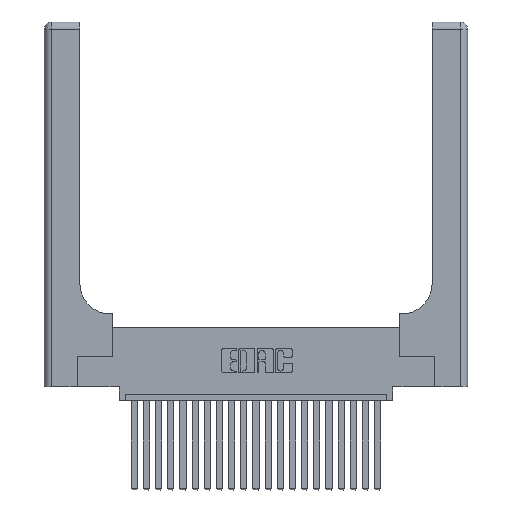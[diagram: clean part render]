
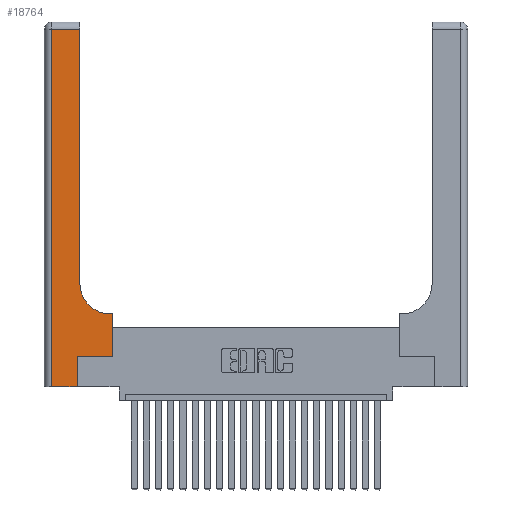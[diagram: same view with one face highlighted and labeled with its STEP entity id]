
A CAD part, top view. The second image highlights one B-rep face of the part: STEP entity #18764.
In plain terms, the highlighted planar face has unit normal (0, 0, 1).
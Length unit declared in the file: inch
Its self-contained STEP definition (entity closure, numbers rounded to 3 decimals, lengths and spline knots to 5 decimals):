
#302 = LINE ( 'NONE', #17518, #9762 ) ;
#973 = CARTESIAN_POINT ( 'NONE',  ( 0., 3., 0.37 ) ) ;
#1057 = VECTOR ( 'NONE', #14050, 39.37008 ) ;
#1203 = DIRECTION ( 'NONE',  ( 0., 1., 0. ) ) ;
#2124 = EDGE_CURVE ( 'NONE', #18836, #19935, #22262, .T. ) ;
#2383 = CARTESIAN_POINT ( 'NONE',  ( 0.2915, 3., 0.37 ) ) ;
#2493 = CARTESIAN_POINT ( 'NONE',  ( 0.5415, 0.85, 0.37 ) ) ;
#2960 = ORIENTED_EDGE ( 'NONE', *, *, #21405, .T. ) ;
#2988 = CARTESIAN_POINT ( 'NONE',  ( 0.06, 2.94, 0.37 ) ) ;
#3067 = CARTESIAN_POINT ( 'NONE',  ( 0.269, 0., 0.37 ) ) ;
#4240 = EDGE_LOOP ( 'NONE', ( #13874, #17022, #5592, #11462, #2960, #12885, #12064, #6538, #22106 ) ) ;
#4311 = CARTESIAN_POINT ( 'NONE',  ( 0.5585, 0.25, 0.37 ) ) ;
#4681 = EDGE_CURVE ( 'NONE', #10254, #18836, #19064, .T. ) ;
#4701 = DIRECTION ( 'NONE',  ( 0., 0., -1. ) ) ;
#5538 = LINE ( 'NONE', #2383, #6696 ) ;
#5592 = ORIENTED_EDGE ( 'NONE', *, *, #2124, .T. ) ;
#5808 = CARTESIAN_POINT ( 'NONE',  ( 0., 0., 0.37 ) ) ;
#6538 = ORIENTED_EDGE ( 'NONE', *, *, #9288, .T. ) ;
#6650 = CARTESIAN_POINT ( 'NONE',  ( 0.06, 0., 0.37 ) ) ;
#6696 = VECTOR ( 'NONE', #20760, 39.37008 ) ;
#6698 = DIRECTION ( 'NONE',  ( -1., 0., 0. ) ) ;
#7909 = DIRECTION ( 'NONE',  ( 0., 1., 0. ) ) ;
#8263 = CARTESIAN_POINT ( 'NONE',  ( 0.06, 3., 0.37 ) ) ;
#9000 = EDGE_CURVE ( 'NONE', #11467, #10174, #20308, .T. ) ;
#9188 = VERTEX_POINT ( 'NONE', #3067 ) ;
#9272 = CARTESIAN_POINT ( 'NONE',  ( 0.5585, 0.6, 0.37 ) ) ;
#9288 = EDGE_CURVE ( 'NONE', #10174, #16898, #20007, .T. ) ;
#9446 = EDGE_CURVE ( 'NONE', #19935, #9188, #17457, .T. ) ;
#9454 = DIRECTION ( 'NONE',  ( 1., 0., 0. ) ) ;
#9687 = VERTEX_POINT ( 'NONE', #17111 ) ;
#9762 = VECTOR ( 'NONE', #1203, 39.37008 ) ;
#10019 = PLANE ( 'NONE',  #14127 ) ;
#10174 = VERTEX_POINT ( 'NONE', #9272 ) ;
#10236 = DIRECTION ( 'NONE',  ( 0., -1., 0. ) ) ;
#10254 = VERTEX_POINT ( 'NONE', #18770 ) ;
#10390 = CARTESIAN_POINT ( 'NONE',  ( 0.5415, 0.6, 0.37 ) ) ;
#11329 = VECTOR ( 'NONE', #10236, 39.37008 ) ;
#11462 = ORIENTED_EDGE ( 'NONE', *, *, #9446, .T. ) ;
#11467 = VERTEX_POINT ( 'NONE', #18810 ) ;
#11528 = EDGE_CURVE ( 'NONE', #16898, #9687, #17903, .T. ) ;
#12064 = ORIENTED_EDGE ( 'NONE', *, *, #9000, .T. ) ;
#12118 = CARTESIAN_POINT ( 'NONE',  ( 0.2915, 0.6, 0.37 ) ) ;
#12885 = ORIENTED_EDGE ( 'NONE', *, *, #23118, .T. ) ;
#13388 = VECTOR ( 'NONE', #9454, 39.37008 ) ;
#13511 = CARTESIAN_POINT ( 'NONE',  ( 0.269, 0.25, 0.37 ) ) ;
#13665 = DIRECTION ( 'NONE',  ( 1., 0., 0. ) ) ;
#13874 = ORIENTED_EDGE ( 'NONE', *, *, #19756, .T. ) ;
#13995 = CARTESIAN_POINT ( 'NONE',  ( 0., 2.94, 0.37 ) ) ;
#14050 = DIRECTION ( 'NONE',  ( -1., 0., 0. ) ) ;
#14127 = AXIS2_PLACEMENT_3D ( 'NONE', #973, #4701, #6698 ) ;
#14134 = VECTOR ( 'NONE', #21318, 39.37008 ) ;
#15199 = CARTESIAN_POINT ( 'NONE',  ( 0.269, 0.25, 0.37 ) ) ;
#15485 = VERTEX_POINT ( 'NONE', #13511 ) ;
#15494 = DIRECTION ( 'NONE',  ( 1., 0., 0. ) ) ;
#15598 = AXIS2_PLACEMENT_3D ( 'NONE', #2493, #22780, #15494 ) ;
#16898 = VERTEX_POINT ( 'NONE', #10390 ) ;
#17022 = ORIENTED_EDGE ( 'NONE', *, *, #4681, .T. ) ;
#17111 = CARTESIAN_POINT ( 'NONE',  ( 0.2915, 0.85, 0.37 ) ) ;
#17457 = LINE ( 'NONE', #5808, #13388 ) ;
#17518 = CARTESIAN_POINT ( 'NONE',  ( 0.269, 0., 0.37 ) ) ;
#17903 = CIRCLE ( 'NONE', #15598, 0.25 ) ;
#18048 = VECTOR ( 'NONE', #13665, 39.37008 ) ;
#18764 = ADVANCED_FACE ( 'NONE', ( #22232 ), #10019, .F. ) ;
#18770 = CARTESIAN_POINT ( 'NONE',  ( 0.2915, 2.94, 0.37 ) ) ;
#18810 = CARTESIAN_POINT ( 'NONE',  ( 0.5585, 0.25, 0.37 ) ) ;
#18836 = VERTEX_POINT ( 'NONE', #2988 ) ;
#19064 = LINE ( 'NONE', #13995, #14134 ) ;
#19756 = EDGE_CURVE ( 'NONE', #9687, #10254, #5538, .T. ) ;
#19935 = VERTEX_POINT ( 'NONE', #6650 ) ;
#20007 = LINE ( 'NONE', #12118, #1057 ) ;
#20029 = VECTOR ( 'NONE', #7909, 39.37008 ) ;
#20308 = LINE ( 'NONE', #4311, #20029 ) ;
#20760 = DIRECTION ( 'NONE',  ( 0., 1., 0. ) ) ;
#21318 = DIRECTION ( 'NONE',  ( -1., 0., 0. ) ) ;
#21405 = EDGE_CURVE ( 'NONE', #9188, #15485, #302, .T. ) ;
#22106 = ORIENTED_EDGE ( 'NONE', *, *, #11528, .T. ) ;
#22232 = FACE_OUTER_BOUND ( 'NONE', #4240, .T. ) ;
#22262 = LINE ( 'NONE', #8263, #11329 ) ;
#22780 = DIRECTION ( 'NONE',  ( 0., 0., -1. ) ) ;
#23118 = EDGE_CURVE ( 'NONE', #15485, #11467, #23456, .T. ) ;
#23456 = LINE ( 'NONE', #15199, #18048 ) ;
